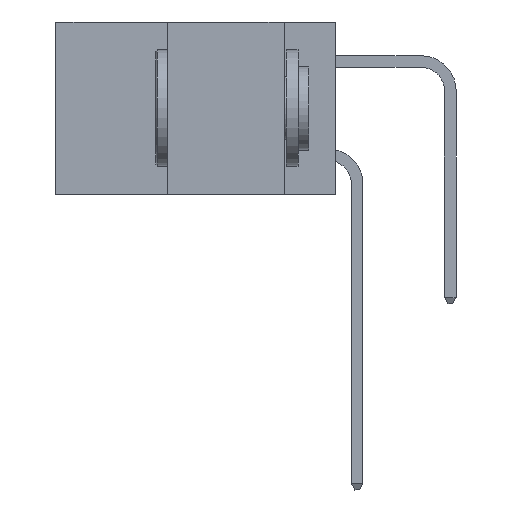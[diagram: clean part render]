
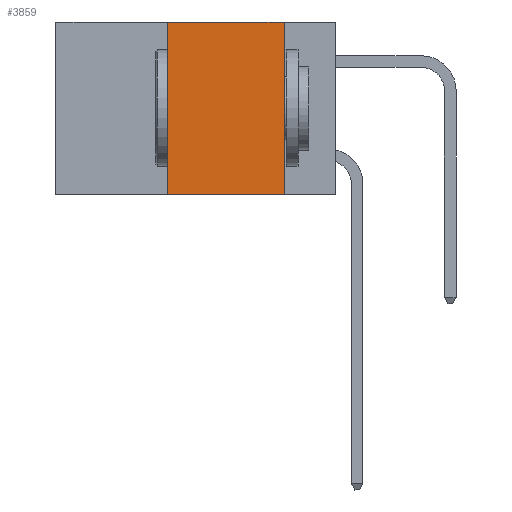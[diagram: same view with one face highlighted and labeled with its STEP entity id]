
A CAD part, left-side view. The second image highlights one B-rep face of the part: STEP entity #3859.
In plain terms, the highlighted planar face has unit normal (-1, 0, 0).
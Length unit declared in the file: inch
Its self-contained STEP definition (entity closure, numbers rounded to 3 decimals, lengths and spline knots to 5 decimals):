
#120 = LINE ( 'NONE', #15590, #9290 ) ;
#839 = VERTEX_POINT ( 'NONE', #7297 ) ;
#897 = CARTESIAN_POINT ( 'NONE',  ( 0., 0.36, -0.37 ) ) ;
#1721 = ORIENTED_EDGE ( 'NONE', *, *, #8643, .F. ) ;
#2449 = DIRECTION ( 'NONE',  ( 0., 0., -1. ) ) ;
#2594 = CARTESIAN_POINT ( 'NONE',  ( 0., 0.11, 0. ) ) ;
#3467 = ORIENTED_EDGE ( 'NONE', *, *, #20831, .T. ) ;
#3859 = ADVANCED_FACE ( 'NONE', ( #17537 ), #9866, .F. ) ;
#4259 = EDGE_LOOP ( 'NONE', ( #18502, #19087, #1721, #3467 ) ) ;
#4377 = VERTEX_POINT ( 'NONE', #897 ) ;
#4892 = EDGE_CURVE ( 'NONE', #9840, #6250, #5738, .T. ) ;
#5738 = LINE ( 'NONE', #7405, #18498 ) ;
#5985 = CARTESIAN_POINT ( 'NONE',  ( 0., 0.6, -0.37 ) ) ;
#6250 = VERTEX_POINT ( 'NONE', #2594 ) ;
#7297 = CARTESIAN_POINT ( 'NONE',  ( 0., 0.11, -0.37 ) ) ;
#7405 = CARTESIAN_POINT ( 'NONE',  ( 0., 0.6, 0. ) ) ;
#7571 = CARTESIAN_POINT ( 'NONE',  ( 0., 0.36, 0. ) ) ;
#8151 = DIRECTION ( 'NONE',  ( 0., 0., -1. ) ) ;
#8643 = EDGE_CURVE ( 'NONE', #4377, #9840, #19628, .T. ) ;
#9290 = VECTOR ( 'NONE', #2449, 39.37008 ) ;
#9467 = AXIS2_PLACEMENT_3D ( 'NONE', #9733, #14722, #8151 ) ;
#9733 = CARTESIAN_POINT ( 'NONE',  ( 0., 0.6, 0. ) ) ;
#9840 = VERTEX_POINT ( 'NONE', #7571 ) ;
#9866 = PLANE ( 'NONE',  #9467 ) ;
#11141 = VECTOR ( 'NONE', #12810, 39.37008 ) ;
#12810 = DIRECTION ( 'NONE',  ( 0., -1., 0. ) ) ;
#13654 = CARTESIAN_POINT ( 'NONE',  ( 0., 0.36, 0. ) ) ;
#14722 = DIRECTION ( 'NONE',  ( 1., 0., 0. ) ) ;
#15388 = EDGE_CURVE ( 'NONE', #6250, #839, #120, .T. ) ;
#15590 = CARTESIAN_POINT ( 'NONE',  ( 0., 0.11, 0. ) ) ;
#16757 = LINE ( 'NONE', #5985, #11141 ) ;
#17537 = FACE_OUTER_BOUND ( 'NONE', #4259, .T. ) ;
#18498 = VECTOR ( 'NONE', #18673, 39.37008 ) ;
#18502 = ORIENTED_EDGE ( 'NONE', *, *, #15388, .F. ) ;
#18673 = DIRECTION ( 'NONE',  ( 0., -1., 0. ) ) ;
#18730 = DIRECTION ( 'NONE',  ( 0., 0., 1. ) ) ;
#19067 = VECTOR ( 'NONE', #18730, 39.37008 ) ;
#19087 = ORIENTED_EDGE ( 'NONE', *, *, #4892, .F. ) ;
#19628 = LINE ( 'NONE', #13654, #19067 ) ;
#20831 = EDGE_CURVE ( 'NONE', #4377, #839, #16757, .T. ) ;
